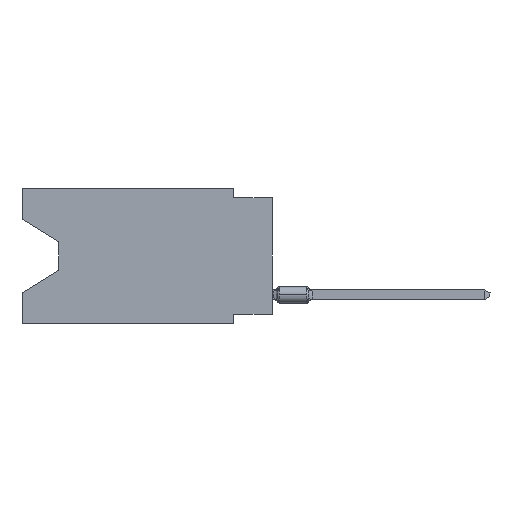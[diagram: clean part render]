
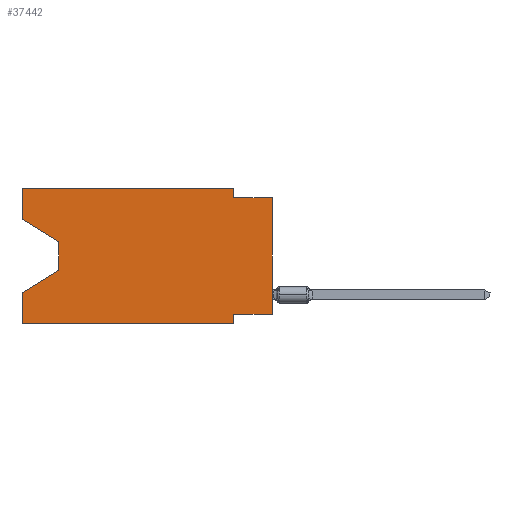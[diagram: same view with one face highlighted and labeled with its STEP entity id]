
A CAD part, left-side view. The second image highlights one B-rep face of the part: STEP entity #37442.
In plain terms, the highlighted planar face has unit normal (-1, 0, 0).
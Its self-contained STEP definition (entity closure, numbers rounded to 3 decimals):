
#64 = EDGE_LOOP ( 'NONE', ( #15542, #36594, #12623, #20288, #18774, #11984, #32417, #10362, #22211, #33755, #40266, #1927 ) ) ;
#95 = CARTESIAN_POINT ( 'NONE',  ( 0., 0., 0. ) ) ;
#406 = EDGE_CURVE ( 'NONE', #17829, #12200, #25078, .T. ) ;
#1927 = ORIENTED_EDGE ( 'NONE', *, *, #34733, .F. ) ;
#2430 = CARTESIAN_POINT ( 'NONE',  ( 0., 0., -8.255 ) ) ;
#2687 = VERTEX_POINT ( 'NONE', #2430 ) ;
#2902 = LINE ( 'NONE', #40474, #6334 ) ;
#3242 = CARTESIAN_POINT ( 'NONE',  ( 0., 16.383, -6.852 ) ) ;
#3758 = VERTEX_POINT ( 'NONE', #3242 ) ;
#4119 = LINE ( 'NONE', #8005, #14144 ) ;
#4467 = DIRECTION ( 'NONE',  ( 0., -1., 0. ) ) ;
#5036 = LINE ( 'NONE', #39924, #14128 ) ;
#5242 = DIRECTION ( 'NONE',  ( 0., 0.855, -0.519 ) ) ;
#5548 = VECTOR ( 'NONE', #4467, 1000. ) ;
#5779 = CARTESIAN_POINT ( 'NONE',  ( 0., 16.383, 0. ) ) ;
#6334 = VECTOR ( 'NONE', #24851, 1000. ) ;
#6350 = VECTOR ( 'NONE', #5242, 1000. ) ;
#7141 = CARTESIAN_POINT ( 'NONE',  ( 0., 13.97, -5.385 ) ) ;
#7773 = VERTEX_POINT ( 'NONE', #20402 ) ;
#8005 = CARTESIAN_POINT ( 'NONE',  ( 0., 0., -8.255 ) ) ;
#8938 = DIRECTION ( 'NONE',  ( 0., 0., 1. ) ) ;
#9970 = EDGE_CURVE ( 'NONE', #20748, #31412, #2902, .T. ) ;
#10362 = ORIENTED_EDGE ( 'NONE', *, *, #19050, .T. ) ;
#10504 = CARTESIAN_POINT ( 'NONE',  ( 0., 0., -0.635 ) ) ;
#11094 = DIRECTION ( 'NONE',  ( 0., 1., 0. ) ) ;
#11234 = LINE ( 'NONE', #36277, #5548 ) ;
#11984 = ORIENTED_EDGE ( 'NONE', *, *, #29379, .F. ) ;
#12079 = VECTOR ( 'NONE', #25344, 1000. ) ;
#12184 = DIRECTION ( 'NONE',  ( 0., 0., -1. ) ) ;
#12200 = VERTEX_POINT ( 'NONE', #7141 ) ;
#12623 = ORIENTED_EDGE ( 'NONE', *, *, #14301, .T. ) ;
#14128 = VECTOR ( 'NONE', #40114, 1000. ) ;
#14144 = VECTOR ( 'NONE', #11094, 1000. ) ;
#14301 = EDGE_CURVE ( 'NONE', #12200, #3758, #30265, .T. ) ;
#15082 = CARTESIAN_POINT ( 'NONE',  ( 0., 16.383, 0. ) ) ;
#15251 = CARTESIAN_POINT ( 'NONE',  ( 0., 16.383, 0. ) ) ;
#15324 = VERTEX_POINT ( 'NONE', #15082 ) ;
#15542 = ORIENTED_EDGE ( 'NONE', *, *, #16770, .T. ) ;
#15908 = EDGE_CURVE ( 'NONE', #2687, #7773, #4119, .T. ) ;
#16770 = EDGE_CURVE ( 'NONE', #35690, #17829, #31545, .T. ) ;
#17104 = DIRECTION ( 'NONE',  ( 1., 0., 0. ) ) ;
#17829 = VERTEX_POINT ( 'NONE', #33439 ) ;
#18774 = ORIENTED_EDGE ( 'NONE', *, *, #38185, .T. ) ;
#18847 = CARTESIAN_POINT ( 'NONE',  ( 0., 16.383, -2.038 ) ) ;
#19050 = EDGE_CURVE ( 'NONE', #2687, #31412, #27616, .T. ) ;
#19256 = DIRECTION ( 'NONE',  ( 0., 0., -1. ) ) ;
#19448 = CARTESIAN_POINT ( 'NONE',  ( 0., 16.383, -2.038 ) ) ;
#19974 = CARTESIAN_POINT ( 'NONE',  ( 0., 16.383, 0. ) ) ;
#20288 = ORIENTED_EDGE ( 'NONE', *, *, #27833, .F. ) ;
#20402 = CARTESIAN_POINT ( 'NONE',  ( 0., 2.54, -8.255 ) ) ;
#20748 = VERTEX_POINT ( 'NONE', #37298 ) ;
#21143 = VECTOR ( 'NONE', #28269, 1000. ) ;
#21181 = DIRECTION ( 'NONE',  ( 0., 0., 1. ) ) ;
#22048 = VERTEX_POINT ( 'NONE', #29494 ) ;
#22056 = CARTESIAN_POINT ( 'NONE',  ( 0., 2.54, 0. ) ) ;
#22211 = ORIENTED_EDGE ( 'NONE', *, *, #9970, .F. ) ;
#22941 = LINE ( 'NONE', #35449, #38842 ) ;
#23777 = VECTOR ( 'NONE', #8938, 1000. ) ;
#23857 = VERTEX_POINT ( 'NONE', #27398 ) ;
#24473 = DIRECTION ( 'NONE',  ( 0., 0., 1. ) ) ;
#24851 = DIRECTION ( 'NONE',  ( 0., -1., 0. ) ) ;
#25078 = LINE ( 'NONE', #31032, #35476 ) ;
#25344 = DIRECTION ( 'NONE',  ( 0., 0., -1. ) ) ;
#27314 = VECTOR ( 'NONE', #24473, 1000. ) ;
#27398 = CARTESIAN_POINT ( 'NONE',  ( 0., 2.54, -8.89 ) ) ;
#27616 = LINE ( 'NONE', #95, #23777 ) ;
#27833 = EDGE_CURVE ( 'NONE', #32628, #3758, #31227, .T. ) ;
#27996 = CARTESIAN_POINT ( 'NONE',  ( 0., 13.97, -5.385 ) ) ;
#28269 = DIRECTION ( 'NONE',  ( 0., -0.855, -0.519 ) ) ;
#29128 = AXIS2_PLACEMENT_3D ( 'NONE', #19974, #17104, #32479 ) ;
#29379 = EDGE_CURVE ( 'NONE', #7773, #23857, #22941, .T. ) ;
#29397 = FACE_OUTER_BOUND ( 'NONE', #64, .T. ) ;
#29494 = CARTESIAN_POINT ( 'NONE',  ( 0., 2.54, 0. ) ) ;
#29592 = PLANE ( 'NONE',  #29128 ) ;
#30265 = LINE ( 'NONE', #27996, #6350 ) ;
#31032 = CARTESIAN_POINT ( 'NONE',  ( 0., 13.97, -3.505 ) ) ;
#31227 = LINE ( 'NONE', #15251, #27314 ) ;
#31412 = VERTEX_POINT ( 'NONE', #10504 ) ;
#31545 = LINE ( 'NONE', #18847, #21143 ) ;
#32417 = ORIENTED_EDGE ( 'NONE', *, *, #15908, .F. ) ;
#32479 = DIRECTION ( 'NONE',  ( 0., 0., -1. ) ) ;
#32628 = VERTEX_POINT ( 'NONE', #40236 ) ;
#33439 = CARTESIAN_POINT ( 'NONE',  ( 0., 13.97, -3.505 ) ) ;
#33755 = ORIENTED_EDGE ( 'NONE', *, *, #37602, .F. ) ;
#34733 = EDGE_CURVE ( 'NONE', #35690, #15324, #37180, .T. ) ;
#35449 = CARTESIAN_POINT ( 'NONE',  ( 0., 2.54, -8.89 ) ) ;
#35476 = VECTOR ( 'NONE', #12184, 1000. ) ;
#35690 = VERTEX_POINT ( 'NONE', #19448 ) ;
#36277 = CARTESIAN_POINT ( 'NONE',  ( 0., 16.383, -8.89 ) ) ;
#36594 = ORIENTED_EDGE ( 'NONE', *, *, #406, .T. ) ;
#37180 = LINE ( 'NONE', #5779, #38376 ) ;
#37257 = LINE ( 'NONE', #22056, #12079 ) ;
#37298 = CARTESIAN_POINT ( 'NONE',  ( 0., 2.54, -0.635 ) ) ;
#37442 = ADVANCED_FACE ( 'NONE', ( #29397 ), #29592, .F. ) ;
#37602 = EDGE_CURVE ( 'NONE', #22048, #20748, #37257, .T. ) ;
#38185 = EDGE_CURVE ( 'NONE', #32628, #23857, #11234, .T. ) ;
#38376 = VECTOR ( 'NONE', #21181, 1000. ) ;
#38772 = EDGE_CURVE ( 'NONE', #15324, #22048, #5036, .T. ) ;
#38842 = VECTOR ( 'NONE', #19256, 1000. ) ;
#39924 = CARTESIAN_POINT ( 'NONE',  ( 0., 16.383, 0. ) ) ;
#40114 = DIRECTION ( 'NONE',  ( 0., -1., 0. ) ) ;
#40236 = CARTESIAN_POINT ( 'NONE',  ( 0., 16.383, -8.89 ) ) ;
#40266 = ORIENTED_EDGE ( 'NONE', *, *, #38772, .F. ) ;
#40474 = CARTESIAN_POINT ( 'NONE',  ( 0., 0., -0.635 ) ) ;
